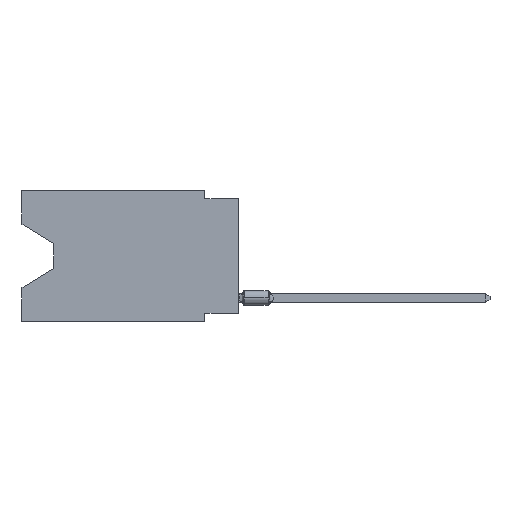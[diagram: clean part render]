
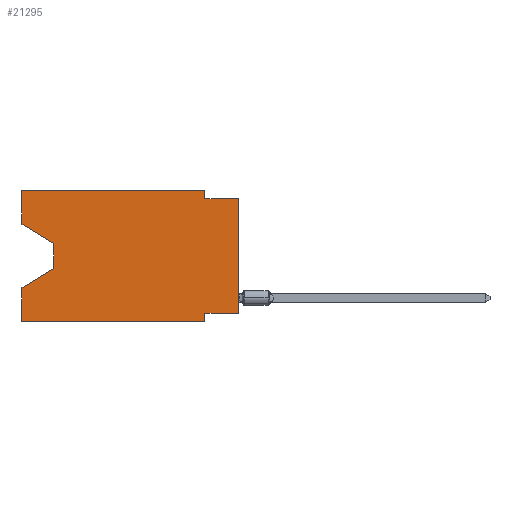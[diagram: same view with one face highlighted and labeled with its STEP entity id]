
A CAD part, left-side view. The second image highlights one B-rep face of the part: STEP entity #21295.
In plain terms, the highlighted planar face has unit normal (-1, 0, 0).
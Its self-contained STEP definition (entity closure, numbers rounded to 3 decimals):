
#1 = VERTEX_POINT ( 'NONE', #2633 ) ;
#196 = CARTESIAN_POINT ( 'NONE',  ( 0., 16.383, 0. ) ) ;
#437 = FACE_OUTER_BOUND ( 'NONE', #22702, .T. ) ;
#473 = DIRECTION ( 'NONE',  ( 0., 0.855, -0.519 ) ) ;
#909 = VECTOR ( 'NONE', #21280, 1000. ) ;
#1130 = VECTOR ( 'NONE', #16164, 1000. ) ;
#1369 = DIRECTION ( 'NONE',  ( 0., 0., 1. ) ) ;
#1478 = CARTESIAN_POINT ( 'NONE',  ( 0., 0., 0. ) ) ;
#1578 = EDGE_CURVE ( 'NONE', #3995, #11539, #3943, .T. ) ;
#1717 = EDGE_CURVE ( 'NONE', #21625, #18281, #15831, .T. ) ;
#1842 = EDGE_CURVE ( 'NONE', #4034, #18281, #20668, .T. ) ;
#1903 = CARTESIAN_POINT ( 'NONE',  ( 0., 16.383, -9.906 ) ) ;
#2137 = VERTEX_POINT ( 'NONE', #6926 ) ;
#2310 = CARTESIAN_POINT ( 'NONE',  ( 0., 0., -0.635 ) ) ;
#2633 = CARTESIAN_POINT ( 'NONE',  ( 0., 0., -9.271 ) ) ;
#3943 = LINE ( 'NONE', #11280, #20892 ) ;
#3995 = VERTEX_POINT ( 'NONE', #5420 ) ;
#4034 = VERTEX_POINT ( 'NONE', #7334 ) ;
#4083 = DIRECTION ( 'NONE',  ( 0., -1., 0. ) ) ;
#4117 = LINE ( 'NONE', #2310, #9934 ) ;
#4575 = VERTEX_POINT ( 'NONE', #22217 ) ;
#5420 = CARTESIAN_POINT ( 'NONE',  ( 0., 13.97, -4.013 ) ) ;
#5738 = ORIENTED_EDGE ( 'NONE', *, *, #1842, .T. ) ;
#6223 = CARTESIAN_POINT ( 'NONE',  ( 0., 2.54, -9.906 ) ) ;
#6258 = EDGE_CURVE ( 'NONE', #1, #18714, #23363, .T. ) ;
#6452 = DIRECTION ( 'NONE',  ( 0., 0., -1. ) ) ;
#6478 = CARTESIAN_POINT ( 'NONE',  ( 0., 16.383, 0. ) ) ;
#6636 = VERTEX_POINT ( 'NONE', #18159 ) ;
#6654 = ORIENTED_EDGE ( 'NONE', *, *, #11568, .T. ) ;
#6850 = VECTOR ( 'NONE', #18203, 1000. ) ;
#6926 = CARTESIAN_POINT ( 'NONE',  ( 0., 2.54, 0. ) ) ;
#6929 = DIRECTION ( 'NONE',  ( 0., -0.855, -0.519 ) ) ;
#7226 = VECTOR ( 'NONE', #10083, 1000. ) ;
#7287 = ORIENTED_EDGE ( 'NONE', *, *, #21470, .F. ) ;
#7334 = CARTESIAN_POINT ( 'NONE',  ( 0., 16.383, -9.906 ) ) ;
#7373 = VECTOR ( 'NONE', #1369, 1000. ) ;
#7763 = ORIENTED_EDGE ( 'NONE', *, *, #23088, .F. ) ;
#7784 = DIRECTION ( 'NONE',  ( 0., 0., -1. ) ) ;
#8023 = CARTESIAN_POINT ( 'NONE',  ( 0., 0., -9.271 ) ) ;
#8509 = CARTESIAN_POINT ( 'NONE',  ( 0., 2.54, -0.635 ) ) ;
#8611 = VECTOR ( 'NONE', #20756, 1000. ) ;
#9179 = CARTESIAN_POINT ( 'NONE',  ( 0., 16.383, 0. ) ) ;
#9289 = ORIENTED_EDGE ( 'NONE', *, *, #1717, .F. ) ;
#9458 = PLANE ( 'NONE',  #22039 ) ;
#9853 = CARTESIAN_POINT ( 'NONE',  ( 0., 13.97, -5.893 ) ) ;
#9934 = VECTOR ( 'NONE', #22268, 1000. ) ;
#10083 = DIRECTION ( 'NONE',  ( 0., 1., 0. ) ) ;
#10334 = EDGE_CURVE ( 'NONE', #18435, #18714, #4117, .T. ) ;
#10799 = ORIENTED_EDGE ( 'NONE', *, *, #6258, .T. ) ;
#11136 = ORIENTED_EDGE ( 'NONE', *, *, #21216, .F. ) ;
#11280 = CARTESIAN_POINT ( 'NONE',  ( 0., 13.97, -4.013 ) ) ;
#11283 = CARTESIAN_POINT ( 'NONE',  ( 0., 16.383, -2.546 ) ) ;
#11539 = VERTEX_POINT ( 'NONE', #9853 ) ;
#11568 = EDGE_CURVE ( 'NONE', #11539, #6636, #22939, .T. ) ;
#11651 = CARTESIAN_POINT ( 'NONE',  ( 0., 2.54, -9.906 ) ) ;
#12007 = LINE ( 'NONE', #16073, #18842 ) ;
#12328 = LINE ( 'NONE', #9179, #1130 ) ;
#12727 = ORIENTED_EDGE ( 'NONE', *, *, #20989, .F. ) ;
#12943 = DIRECTION ( 'NONE',  ( 0., 0., -1. ) ) ;
#14775 = ORIENTED_EDGE ( 'NONE', *, *, #16136, .T. ) ;
#15098 = CARTESIAN_POINT ( 'NONE',  ( 0., 2.54, 0. ) ) ;
#15521 = VECTOR ( 'NONE', #6452, 1000. ) ;
#15831 = LINE ( 'NONE', #6223, #15521 ) ;
#16073 = CARTESIAN_POINT ( 'NONE',  ( 0., 16.383, -2.546 ) ) ;
#16136 = EDGE_CURVE ( 'NONE', #22938, #3995, #12007, .T. ) ;
#16164 = DIRECTION ( 'NONE',  ( 0., 0., 1. ) ) ;
#16483 = VECTOR ( 'NONE', #4083, 1000. ) ;
#16638 = LINE ( 'NONE', #15098, #6850 ) ;
#16770 = DIRECTION ( 'NONE',  ( 1., 0., 0. ) ) ;
#16909 = VECTOR ( 'NONE', #473, 1000. ) ;
#16926 = CARTESIAN_POINT ( 'NONE',  ( 0., 13.97, -5.893 ) ) ;
#17019 = CARTESIAN_POINT ( 'NONE',  ( 0., 16.383, 0. ) ) ;
#17031 = EDGE_CURVE ( 'NONE', #2137, #18435, #16638, .T. ) ;
#18159 = CARTESIAN_POINT ( 'NONE',  ( 0., 16.383, -7.36 ) ) ;
#18203 = DIRECTION ( 'NONE',  ( 0., 0., -1. ) ) ;
#18281 = VERTEX_POINT ( 'NONE', #11651 ) ;
#18435 = VERTEX_POINT ( 'NONE', #8509 ) ;
#18709 = LINE ( 'NONE', #8023, #7226 ) ;
#18714 = VERTEX_POINT ( 'NONE', #22181 ) ;
#18783 = ORIENTED_EDGE ( 'NONE', *, *, #17031, .F. ) ;
#18842 = VECTOR ( 'NONE', #6929, 1000. ) ;
#18886 = ORIENTED_EDGE ( 'NONE', *, *, #10334, .F. ) ;
#20668 = LINE ( 'NONE', #1903, #16483 ) ;
#20756 = DIRECTION ( 'NONE',  ( 0., -1., 0. ) ) ;
#20892 = VECTOR ( 'NONE', #12943, 1000. ) ;
#20989 = EDGE_CURVE ( 'NONE', #22938, #4575, #21035, .T. ) ;
#21035 = LINE ( 'NONE', #6478, #909 ) ;
#21216 = EDGE_CURVE ( 'NONE', #4575, #2137, #22447, .T. ) ;
#21280 = DIRECTION ( 'NONE',  ( 0., 0., 1. ) ) ;
#21295 = ADVANCED_FACE ( 'NONE', ( #437 ), #9458, .F. ) ;
#21470 = EDGE_CURVE ( 'NONE', #4034, #6636, #12328, .T. ) ;
#21625 = VERTEX_POINT ( 'NONE', #22418 ) ;
#22039 = AXIS2_PLACEMENT_3D ( 'NONE', #196, #16770, #7784 ) ;
#22181 = CARTESIAN_POINT ( 'NONE',  ( 0., 0., -0.635 ) ) ;
#22217 = CARTESIAN_POINT ( 'NONE',  ( 0., 16.383, 0. ) ) ;
#22268 = DIRECTION ( 'NONE',  ( 0., -1., 0. ) ) ;
#22418 = CARTESIAN_POINT ( 'NONE',  ( 0., 2.54, -9.271 ) ) ;
#22447 = LINE ( 'NONE', #17019, #8611 ) ;
#22702 = EDGE_LOOP ( 'NONE', ( #14775, #23679, #6654, #7287, #5738, #9289, #7763, #10799, #18886, #18783, #11136, #12727 ) ) ;
#22938 = VERTEX_POINT ( 'NONE', #11283 ) ;
#22939 = LINE ( 'NONE', #16926, #16909 ) ;
#23088 = EDGE_CURVE ( 'NONE', #1, #21625, #18709, .T. ) ;
#23363 = LINE ( 'NONE', #1478, #7373 ) ;
#23679 = ORIENTED_EDGE ( 'NONE', *, *, #1578, .T. ) ;
